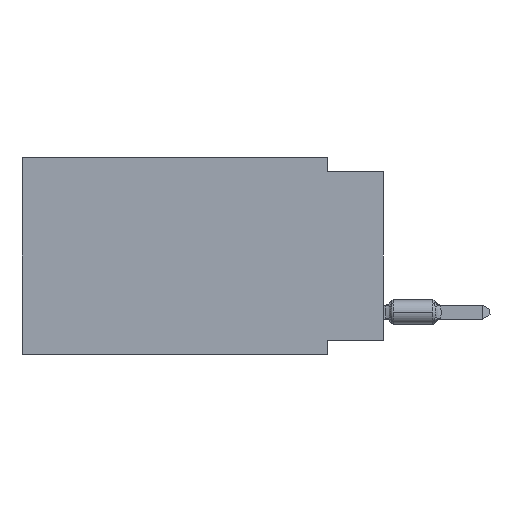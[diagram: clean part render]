
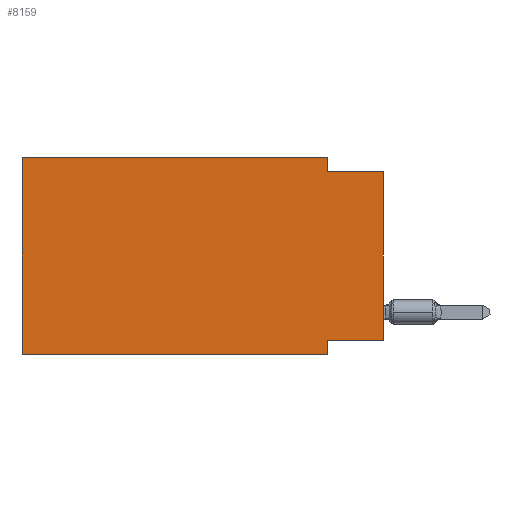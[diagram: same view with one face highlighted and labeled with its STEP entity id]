
A CAD part, left-side view. The second image highlights one B-rep face of the part: STEP entity #8159.
In plain terms, the highlighted planar face has unit normal (-1, 0, 0).
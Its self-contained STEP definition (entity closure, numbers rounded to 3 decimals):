
#64 = DIRECTION ( 'NONE',  ( 0., 0., 1. ) ) ;
#1270 = DIRECTION ( 'NONE',  ( 0., -1., 0. ) ) ;
#1555 = CARTESIAN_POINT ( 'NONE',  ( 0., 2.54, -8.89 ) ) ;
#1822 = VECTOR ( 'NONE', #15112, 1000. ) ;
#2104 = ORIENTED_EDGE ( 'NONE', *, *, #14615, .F. ) ;
#2490 = ORIENTED_EDGE ( 'NONE', *, *, #16162, .F. ) ;
#2503 = LINE ( 'NONE', #10771, #12934 ) ;
#2890 = CARTESIAN_POINT ( 'NONE',  ( 0., 16.383, -8.89 ) ) ;
#2982 = VERTEX_POINT ( 'NONE', #17985 ) ;
#2995 = CARTESIAN_POINT ( 'NONE',  ( 0., 0., 0. ) ) ;
#3620 = EDGE_CURVE ( 'NONE', #14754, #12360, #8620, .T. ) ;
#4028 = ORIENTED_EDGE ( 'NONE', *, *, #6424, .F. ) ;
#4180 = ORIENTED_EDGE ( 'NONE', *, *, #13331, .F. ) ;
#4200 = DIRECTION ( 'NONE',  ( 0., 0., -1. ) ) ;
#4236 = EDGE_LOOP ( 'NONE', ( #17254, #4180, #7932, #9088, #2104, #7970, #4028, #2490 ) ) ;
#4443 = CARTESIAN_POINT ( 'NONE',  ( 0., 2.54, -8.255 ) ) ;
#4581 = LINE ( 'NONE', #5764, #6297 ) ;
#4605 = CARTESIAN_POINT ( 'NONE',  ( 0., 2.54, 0. ) ) ;
#5074 = DIRECTION ( 'NONE',  ( 0., 1., 0. ) ) ;
#5252 = VERTEX_POINT ( 'NONE', #5668 ) ;
#5438 = DIRECTION ( 'NONE',  ( 0., 0., 1. ) ) ;
#5668 = CARTESIAN_POINT ( 'NONE',  ( 0., 2.54, -0.635 ) ) ;
#5764 = CARTESIAN_POINT ( 'NONE',  ( 0., 2.54, -8.89 ) ) ;
#6297 = VECTOR ( 'NONE', #4200, 1000. ) ;
#6424 = EDGE_CURVE ( 'NONE', #13111, #12360, #4581, .T. ) ;
#7932 = ORIENTED_EDGE ( 'NONE', *, *, #10327, .F. ) ;
#7970 = ORIENTED_EDGE ( 'NONE', *, *, #3620, .T. ) ;
#8159 = ADVANCED_FACE ( 'NONE', ( #9667 ), #17046, .F. ) ;
#8216 = VECTOR ( 'NONE', #17261, 1000. ) ;
#8341 = EDGE_CURVE ( 'NONE', #9155, #13691, #17230, .T. ) ;
#8620 = LINE ( 'NONE', #10290, #11301 ) ;
#8902 = CARTESIAN_POINT ( 'NONE',  ( 0., 0., -0.635 ) ) ;
#8905 = VECTOR ( 'NONE', #64, 1000. ) ;
#9088 = ORIENTED_EDGE ( 'NONE', *, *, #8341, .F. ) ;
#9109 = LINE ( 'NONE', #4605, #1822 ) ;
#9155 = VERTEX_POINT ( 'NONE', #14038 ) ;
#9234 = VERTEX_POINT ( 'NONE', #8902 ) ;
#9278 = CARTESIAN_POINT ( 'NONE',  ( 0., 16.383, 0. ) ) ;
#9667 = FACE_OUTER_BOUND ( 'NONE', #4236, .T. ) ;
#9771 = DIRECTION ( 'NONE',  ( 0., -1., 0. ) ) ;
#10290 = CARTESIAN_POINT ( 'NONE',  ( 0., 16.383, -8.89 ) ) ;
#10327 = EDGE_CURVE ( 'NONE', #13691, #5252, #9109, .T. ) ;
#10771 = CARTESIAN_POINT ( 'NONE',  ( 0., 16.383, 0. ) ) ;
#11061 = DIRECTION ( 'NONE',  ( 0., 0., -1. ) ) ;
#11142 = EDGE_CURVE ( 'NONE', #2982, #9234, #19368, .T. ) ;
#11277 = CARTESIAN_POINT ( 'NONE',  ( 0., 0., -0.635 ) ) ;
#11301 = VECTOR ( 'NONE', #1270, 1000. ) ;
#12360 = VERTEX_POINT ( 'NONE', #1555 ) ;
#12518 = DIRECTION ( 'NONE',  ( 1., 0., 0. ) ) ;
#12601 = LINE ( 'NONE', #18501, #16764 ) ;
#12934 = VECTOR ( 'NONE', #5438, 1000. ) ;
#13111 = VERTEX_POINT ( 'NONE', #4443 ) ;
#13331 = EDGE_CURVE ( 'NONE', #5252, #9234, #18542, .T. ) ;
#13691 = VERTEX_POINT ( 'NONE', #14192 ) ;
#14038 = CARTESIAN_POINT ( 'NONE',  ( 0., 16.383, 0. ) ) ;
#14192 = CARTESIAN_POINT ( 'NONE',  ( 0., 2.54, 0. ) ) ;
#14615 = EDGE_CURVE ( 'NONE', #14754, #9155, #2503, .T. ) ;
#14754 = VERTEX_POINT ( 'NONE', #2890 ) ;
#15110 = AXIS2_PLACEMENT_3D ( 'NONE', #9278, #12518, #11061 ) ;
#15112 = DIRECTION ( 'NONE',  ( 0., 0., -1. ) ) ;
#16154 = CARTESIAN_POINT ( 'NONE',  ( 0., 16.383, 0. ) ) ;
#16162 = EDGE_CURVE ( 'NONE', #2982, #13111, #12601, .T. ) ;
#16243 = VECTOR ( 'NONE', #9771, 1000. ) ;
#16764 = VECTOR ( 'NONE', #5074, 1000. ) ;
#17046 = PLANE ( 'NONE',  #15110 ) ;
#17230 = LINE ( 'NONE', #16154, #16243 ) ;
#17254 = ORIENTED_EDGE ( 'NONE', *, *, #11142, .T. ) ;
#17261 = DIRECTION ( 'NONE',  ( 0., -1., 0. ) ) ;
#17985 = CARTESIAN_POINT ( 'NONE',  ( 0., 0., -8.255 ) ) ;
#18501 = CARTESIAN_POINT ( 'NONE',  ( 0., 0., -8.255 ) ) ;
#18542 = LINE ( 'NONE', #11277, #8216 ) ;
#19368 = LINE ( 'NONE', #2995, #8905 ) ;
